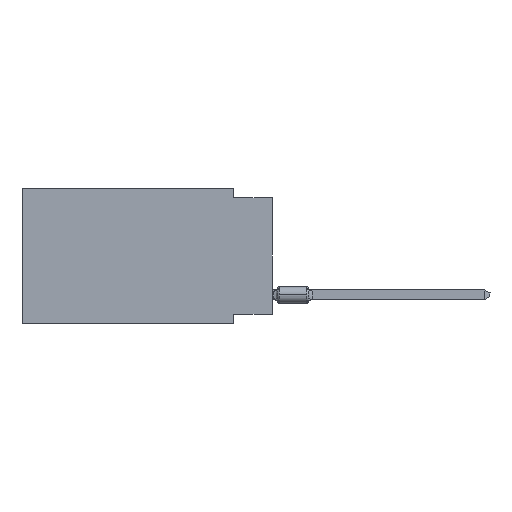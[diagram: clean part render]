
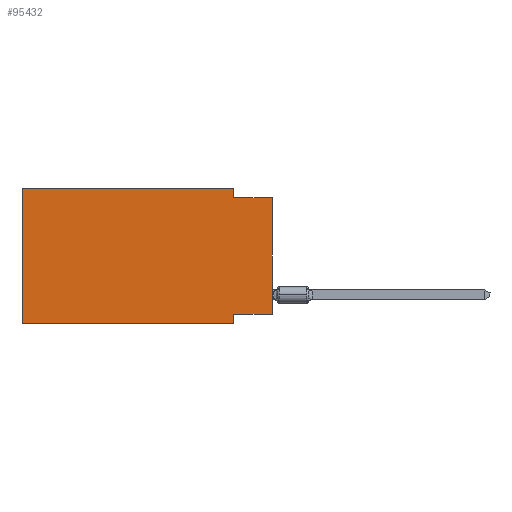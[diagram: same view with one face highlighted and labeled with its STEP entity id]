
A CAD part, left-side view. The second image highlights one B-rep face of the part: STEP entity #95432.
In plain terms, the highlighted planar face has unit normal (-1, 0, 0).
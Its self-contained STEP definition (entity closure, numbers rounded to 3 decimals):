
#2167 = DIRECTION ( 'NONE',  ( 1., 0., 0. ) ) ;
#3141 = EDGE_CURVE ( 'NONE', #52928, #11052, #13413, .T. ) ;
#7027 = CARTESIAN_POINT ( 'NONE',  ( 0., 16.383, -8.89 ) ) ;
#10715 = LINE ( 'NONE', #34589, #60175 ) ;
#11052 = VERTEX_POINT ( 'NONE', #26374 ) ;
#12192 = DIRECTION ( 'NONE',  ( 0., 0., -1. ) ) ;
#13413 = LINE ( 'NONE', #61679, #68174 ) ;
#13909 = EDGE_CURVE ( 'NONE', #68910, #63545, #52355, .T. ) ;
#14137 = DIRECTION ( 'NONE',  ( 0., -1., 0. ) ) ;
#14904 = CARTESIAN_POINT ( 'NONE',  ( 0., 0., -0.635 ) ) ;
#16144 = CARTESIAN_POINT ( 'NONE',  ( 0., 2.54, -8.89 ) ) ;
#17726 = DIRECTION ( 'NONE',  ( 0., 0., 1. ) ) ;
#18692 = EDGE_CURVE ( 'NONE', #88507, #63545, #31916, .T. ) ;
#18837 = VERTEX_POINT ( 'NONE', #33534 ) ;
#21552 = CARTESIAN_POINT ( 'NONE',  ( 0., 2.54, 0. ) ) ;
#22743 = ORIENTED_EDGE ( 'NONE', *, *, #65992, .F. ) ;
#26019 = DIRECTION ( 'NONE',  ( 0., 0., -1. ) ) ;
#26374 = CARTESIAN_POINT ( 'NONE',  ( 0., 2.54, -0.635 ) ) ;
#26901 = VECTOR ( 'NONE', #17726, 1000. ) ;
#26934 = CARTESIAN_POINT ( 'NONE',  ( 0., 0., 0. ) ) ;
#31397 = DIRECTION ( 'NONE',  ( 0., -1., 0. ) ) ;
#31916 = LINE ( 'NONE', #47124, #92904 ) ;
#32764 = AXIS2_PLACEMENT_3D ( 'NONE', #84563, #2167, #26019 ) ;
#32792 = CARTESIAN_POINT ( 'NONE',  ( 0., 16.383, 0. ) ) ;
#33180 = EDGE_CURVE ( 'NONE', #11052, #80933, #54273, .T. ) ;
#33534 = CARTESIAN_POINT ( 'NONE',  ( 0., 16.383, 0. ) ) ;
#34589 = CARTESIAN_POINT ( 'NONE',  ( 0., 0., -8.255 ) ) ;
#36085 = DIRECTION ( 'NONE',  ( 0., 0., 1. ) ) ;
#36610 = LINE ( 'NONE', #69655, #65810 ) ;
#37402 = VECTOR ( 'NONE', #65837, 1000. ) ;
#41732 = ORIENTED_EDGE ( 'NONE', *, *, #90143, .T. ) ;
#43743 = LINE ( 'NONE', #26934, #26901 ) ;
#43986 = LINE ( 'NONE', #32792, #37402 ) ;
#45768 = EDGE_LOOP ( 'NONE', ( #41732, #101861, #52820, #22743, #58574, #74052, #51558, #51891 ) ) ;
#47124 = CARTESIAN_POINT ( 'NONE',  ( 0., 16.383, -8.89 ) ) ;
#49664 = VECTOR ( 'NONE', #14137, 1000. ) ;
#49885 = CARTESIAN_POINT ( 'NONE',  ( 0., 0., -8.255 ) ) ;
#50859 = EDGE_CURVE ( 'NONE', #75096, #68910, #10715, .T. ) ;
#51558 = ORIENTED_EDGE ( 'NONE', *, *, #13909, .F. ) ;
#51891 = ORIENTED_EDGE ( 'NONE', *, *, #50859, .F. ) ;
#52355 = LINE ( 'NONE', #69664, #80101 ) ;
#52820 = ORIENTED_EDGE ( 'NONE', *, *, #3141, .F. ) ;
#52928 = VERTEX_POINT ( 'NONE', #21552 ) ;
#54273 = LINE ( 'NONE', #96019, #49664 ) ;
#58574 = ORIENTED_EDGE ( 'NONE', *, *, #100038, .F. ) ;
#60175 = VECTOR ( 'NONE', #92606, 1000. ) ;
#61679 = CARTESIAN_POINT ( 'NONE',  ( 0., 2.54, 0. ) ) ;
#63545 = VERTEX_POINT ( 'NONE', #16144 ) ;
#65810 = VECTOR ( 'NONE', #36085, 1000. ) ;
#65837 = DIRECTION ( 'NONE',  ( 0., -1., 0. ) ) ;
#65992 = EDGE_CURVE ( 'NONE', #18837, #52928, #43986, .T. ) ;
#68174 = VECTOR ( 'NONE', #103417, 1000. ) ;
#68910 = VERTEX_POINT ( 'NONE', #82946 ) ;
#69655 = CARTESIAN_POINT ( 'NONE',  ( 0., 16.383, 0. ) ) ;
#69664 = CARTESIAN_POINT ( 'NONE',  ( 0., 2.54, -8.89 ) ) ;
#74052 = ORIENTED_EDGE ( 'NONE', *, *, #18692, .T. ) ;
#75096 = VERTEX_POINT ( 'NONE', #49885 ) ;
#80101 = VECTOR ( 'NONE', #12192, 1000. ) ;
#80933 = VERTEX_POINT ( 'NONE', #14904 ) ;
#82021 = PLANE ( 'NONE',  #32764 ) ;
#82946 = CARTESIAN_POINT ( 'NONE',  ( 0., 2.54, -8.255 ) ) ;
#84563 = CARTESIAN_POINT ( 'NONE',  ( 0., 16.383, 0. ) ) ;
#88507 = VERTEX_POINT ( 'NONE', #7027 ) ;
#90143 = EDGE_CURVE ( 'NONE', #75096, #80933, #43743, .T. ) ;
#92606 = DIRECTION ( 'NONE',  ( 0., 1., 0. ) ) ;
#92704 = FACE_OUTER_BOUND ( 'NONE', #45768, .T. ) ;
#92904 = VECTOR ( 'NONE', #31397, 1000. ) ;
#95432 = ADVANCED_FACE ( 'NONE', ( #92704 ), #82021, .F. ) ;
#96019 = CARTESIAN_POINT ( 'NONE',  ( 0., 0., -0.635 ) ) ;
#100038 = EDGE_CURVE ( 'NONE', #88507, #18837, #36610, .T. ) ;
#101861 = ORIENTED_EDGE ( 'NONE', *, *, #33180, .F. ) ;
#103417 = DIRECTION ( 'NONE',  ( 0., 0., -1. ) ) ;
